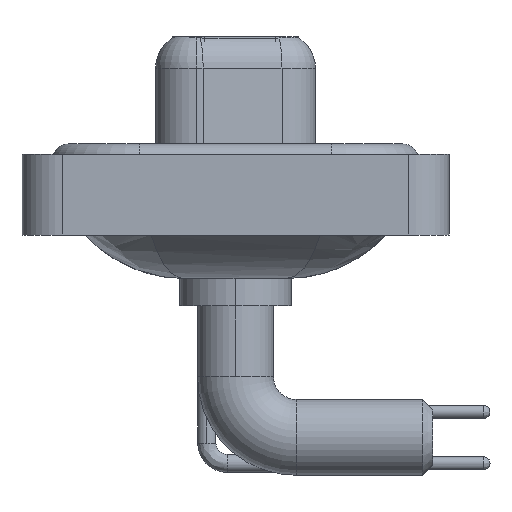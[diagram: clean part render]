
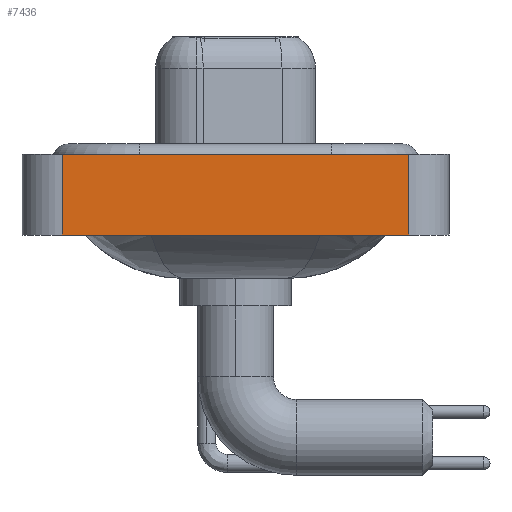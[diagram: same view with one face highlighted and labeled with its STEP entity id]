
A CAD part, left-side view. The second image highlights one B-rep face of the part: STEP entity #7436.
In plain terms, the highlighted planar face has unit normal (-1, 0, 0).
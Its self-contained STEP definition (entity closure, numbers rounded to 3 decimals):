
#247 = EDGE_CURVE ( 'NONE', #10981, #19252, #11628, .T. ) ;
#414 = PLANE ( 'NONE',  #15188 ) ;
#769 = CARTESIAN_POINT ( 'NONE',  ( -7.35, -8.55, -3.6 ) ) ;
#905 = CARTESIAN_POINT ( 'NONE',  ( -7.35, -8.55, 0.4 ) ) ;
#1033 = EDGE_CURVE ( 'NONE', #15861, #19252, #6299, .T. ) ;
#1867 = CARTESIAN_POINT ( 'NONE',  ( -7.35, -8.55, -3.6 ) ) ;
#2390 = FACE_OUTER_BOUND ( 'NONE', #8132, .T. ) ;
#2904 = DIRECTION ( 'NONE',  ( 0., -1., 0. ) ) ;
#3091 = VECTOR ( 'NONE', #22192, 1000. ) ;
#3464 = CARTESIAN_POINT ( 'NONE',  ( -7.35, 8.55, 0.4 ) ) ;
#3826 = LINE ( 'NONE', #10801, #7832 ) ;
#3974 = ORIENTED_EDGE ( 'NONE', *, *, #9514, .F. ) ;
#4466 = DIRECTION ( 'NONE',  ( 0., 0., 1. ) ) ;
#5463 = ORIENTED_EDGE ( 'NONE', *, *, #247, .F. ) ;
#5528 = DIRECTION ( 'NONE',  ( 0., -1., 0. ) ) ;
#5671 = ORIENTED_EDGE ( 'NONE', *, *, #1033, .T. ) ;
#6299 = LINE ( 'NONE', #15187, #3091 ) ;
#7436 = ADVANCED_FACE ( 'NONE', ( #2390 ), #414, .T. ) ;
#7832 = VECTOR ( 'NONE', #5528, 1000. ) ;
#8132 = EDGE_LOOP ( 'NONE', ( #5671, #5463, #3974, #17851 ) ) ;
#9514 = EDGE_CURVE ( 'NONE', #10255, #10981, #15425, .T. ) ;
#10255 = VERTEX_POINT ( 'NONE', #16885 ) ;
#10801 = CARTESIAN_POINT ( 'NONE',  ( -7.35, -8.55, -3.6 ) ) ;
#10981 = VERTEX_POINT ( 'NONE', #3464 ) ;
#11628 = LINE ( 'NONE', #15441, #18847 ) ;
#15187 = CARTESIAN_POINT ( 'NONE',  ( -7.35, -8.55, -3.6 ) ) ;
#15188 = AXIS2_PLACEMENT_3D ( 'NONE', #769, #16178, #4466 ) ;
#15425 = LINE ( 'NONE', #18409, #21314 ) ;
#15441 = CARTESIAN_POINT ( 'NONE',  ( -7.35, -8.55, 0.4 ) ) ;
#15861 = VERTEX_POINT ( 'NONE', #1867 ) ;
#16178 = DIRECTION ( 'NONE',  ( -1., 0., 0. ) ) ;
#16885 = CARTESIAN_POINT ( 'NONE',  ( -7.35, 8.55, -3.6 ) ) ;
#17510 = EDGE_CURVE ( 'NONE', #10255, #15861, #3826, .T. ) ;
#17851 = ORIENTED_EDGE ( 'NONE', *, *, #17510, .T. ) ;
#18409 = CARTESIAN_POINT ( 'NONE',  ( -7.35, 8.55, -3.6 ) ) ;
#18847 = VECTOR ( 'NONE', #2904, 1000. ) ;
#19252 = VERTEX_POINT ( 'NONE', #905 ) ;
#20489 = DIRECTION ( 'NONE',  ( 0., 0., 1. ) ) ;
#21314 = VECTOR ( 'NONE', #20489, 1000. ) ;
#22192 = DIRECTION ( 'NONE',  ( 0., 0., 1. ) ) ;
